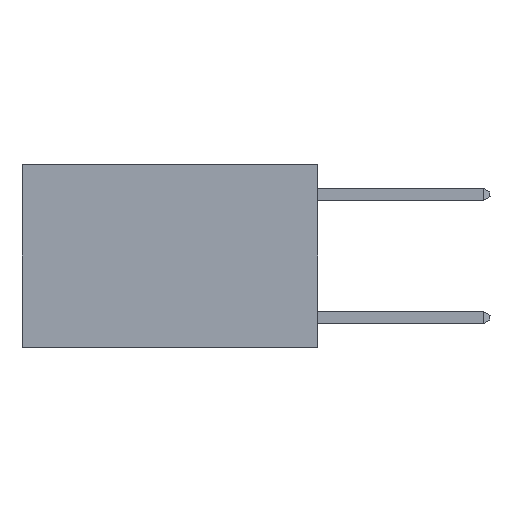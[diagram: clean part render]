
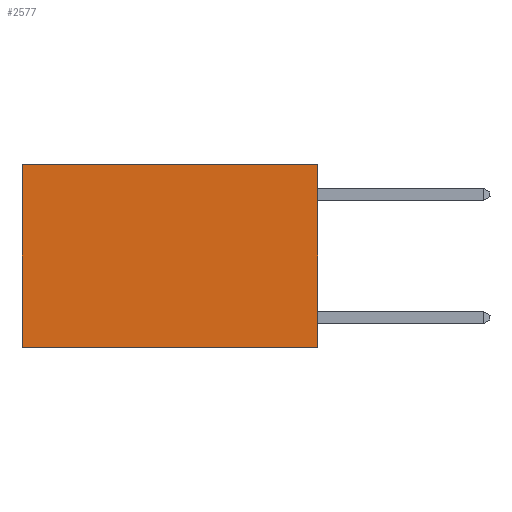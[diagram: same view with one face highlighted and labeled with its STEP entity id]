
A CAD part, left-side view. The second image highlights one B-rep face of the part: STEP entity #2577.
In plain terms, the highlighted planar face has unit normal (-1, 0, 0).
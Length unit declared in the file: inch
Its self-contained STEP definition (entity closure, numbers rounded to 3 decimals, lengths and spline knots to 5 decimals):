
#49 = ORIENTED_EDGE ( 'NONE', *, *, #20241, .T. ) ;
#1136 = LINE ( 'NONE', #6135, #15782 ) ;
#2577 = ADVANCED_FACE ( 'NONE', ( #20078 ), #9696, .F. ) ;
#3368 = CARTESIAN_POINT ( 'NONE',  ( 0.2625, 0., 0. ) ) ;
#4408 = DIRECTION ( 'NONE',  ( 0., 1., 0. ) ) ;
#4422 = EDGE_LOOP ( 'NONE', ( #11784, #8669, #14718, #49 ) ) ;
#4771 = EDGE_CURVE ( 'NONE', #13917, #5692, #1136, .T. ) ;
#5007 = VECTOR ( 'NONE', #4408, 39.37008 ) ;
#5215 = CARTESIAN_POINT ( 'NONE',  ( 0.2625, 0.6, 0. ) ) ;
#5692 = VERTEX_POINT ( 'NONE', #16519 ) ;
#6135 = CARTESIAN_POINT ( 'NONE',  ( 0.2625, 0., -0.37 ) ) ;
#6827 = VECTOR ( 'NONE', #10298, 39.37008 ) ;
#8669 = ORIENTED_EDGE ( 'NONE', *, *, #4771, .F. ) ;
#9696 = PLANE ( 'NONE',  #17080 ) ;
#10072 = CARTESIAN_POINT ( 'NONE',  ( 0.2625, 0., 0. ) ) ;
#10298 = DIRECTION ( 'NONE',  ( 0., 0., -1. ) ) ;
#10551 = VERTEX_POINT ( 'NONE', #20622 ) ;
#10553 = CARTESIAN_POINT ( 'NONE',  ( 0.2625, 0., -0.37 ) ) ;
#10678 = DIRECTION ( 'NONE',  ( 0., 0., -1. ) ) ;
#11784 = ORIENTED_EDGE ( 'NONE', *, *, #19976, .T. ) ;
#13917 = VERTEX_POINT ( 'NONE', #10553 ) ;
#14718 = ORIENTED_EDGE ( 'NONE', *, *, #20407, .F. ) ;
#15777 = LINE ( 'NONE', #3368, #6827 ) ;
#15782 = VECTOR ( 'NONE', #19919, 39.37008 ) ;
#16519 = CARTESIAN_POINT ( 'NONE',  ( 0.2625, 0.6, -0.37 ) ) ;
#17080 = AXIS2_PLACEMENT_3D ( 'NONE', #22146, #18131, #20307 ) ;
#17361 = VECTOR ( 'NONE', #10678, 39.37008 ) ;
#18131 = DIRECTION ( 'NONE',  ( 1., 0., 0. ) ) ;
#19034 = VERTEX_POINT ( 'NONE', #19986 ) ;
#19919 = DIRECTION ( 'NONE',  ( 0., 1., 0. ) ) ;
#19976 = EDGE_CURVE ( 'NONE', #19034, #5692, #20824, .T. ) ;
#19986 = CARTESIAN_POINT ( 'NONE',  ( 0.2625, 0.6, 0. ) ) ;
#20012 = LINE ( 'NONE', #10072, #5007 ) ;
#20078 = FACE_OUTER_BOUND ( 'NONE', #4422, .T. ) ;
#20241 = EDGE_CURVE ( 'NONE', #10551, #19034, #20012, .T. ) ;
#20307 = DIRECTION ( 'NONE',  ( 0., 0., -1. ) ) ;
#20407 = EDGE_CURVE ( 'NONE', #10551, #13917, #15777, .T. ) ;
#20622 = CARTESIAN_POINT ( 'NONE',  ( 0.2625, 0., 0. ) ) ;
#20824 = LINE ( 'NONE', #5215, #17361 ) ;
#22146 = CARTESIAN_POINT ( 'NONE',  ( 0.2625, 0., 0. ) ) ;
